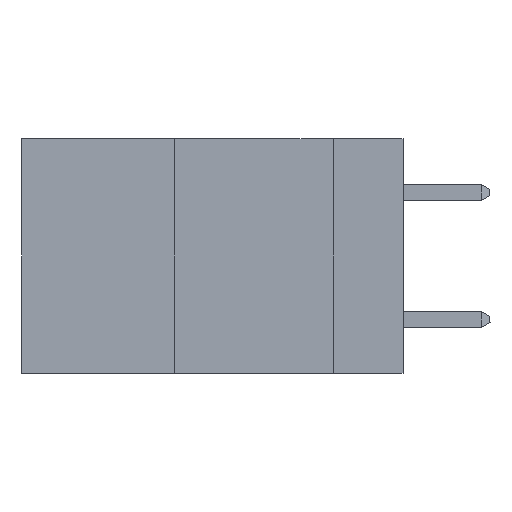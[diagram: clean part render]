
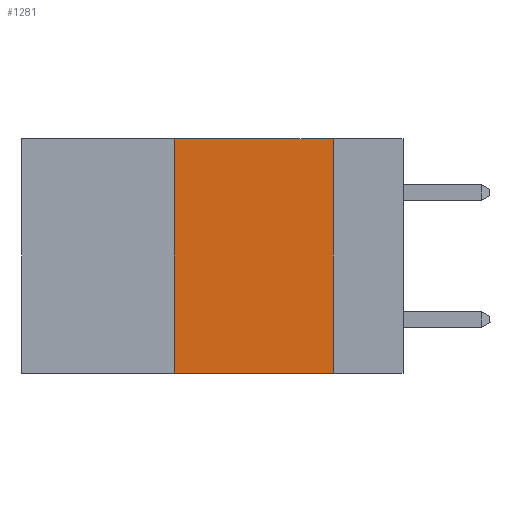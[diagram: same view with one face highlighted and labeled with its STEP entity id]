
A CAD part, left-side view. The second image highlights one B-rep face of the part: STEP entity #1281.
In plain terms, the highlighted planar face has unit normal (-1, 0, 0).
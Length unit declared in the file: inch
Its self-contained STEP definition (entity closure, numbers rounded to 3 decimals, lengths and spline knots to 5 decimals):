
#182 = CARTESIAN_POINT ( 'NONE',  ( 0., 0.11, -0.37 ) ) ;
#314 = DIRECTION ( 'NONE',  ( 0., -1., 0. ) ) ;
#464 = VERTEX_POINT ( 'NONE', #15426 ) ;
#518 = VECTOR ( 'NONE', #14986, 39.37008 ) ;
#656 = FACE_OUTER_BOUND ( 'NONE', #2852, .T. ) ;
#858 = AXIS2_PLACEMENT_3D ( 'NONE', #4481, #3514, #11802 ) ;
#1281 = ADVANCED_FACE ( 'NONE', ( #656 ), #10630, .F. ) ;
#2833 = VERTEX_POINT ( 'NONE', #182 ) ;
#2852 = EDGE_LOOP ( 'NONE', ( #10899, #14367, #5360, #5724 ) ) ;
#3158 = CARTESIAN_POINT ( 'NONE',  ( 0., 0.6, 0. ) ) ;
#3514 = DIRECTION ( 'NONE',  ( 1., 0., 0. ) ) ;
#4474 = EDGE_CURVE ( 'NONE', #464, #9095, #7384, .T. ) ;
#4481 = CARTESIAN_POINT ( 'NONE',  ( 0., 0.6, 0. ) ) ;
#4850 = CARTESIAN_POINT ( 'NONE',  ( 0., 0.36, -0.37 ) ) ;
#5073 = LINE ( 'NONE', #11168, #7831 ) ;
#5360 = ORIENTED_EDGE ( 'NONE', *, *, #6308, .F. ) ;
#5724 = ORIENTED_EDGE ( 'NONE', *, *, #8978, .T. ) ;
#6308 = EDGE_CURVE ( 'NONE', #8228, #464, #13209, .T. ) ;
#6745 = CARTESIAN_POINT ( 'NONE',  ( 0., 0.36, 0. ) ) ;
#7384 = LINE ( 'NONE', #3158, #10164 ) ;
#7831 = VECTOR ( 'NONE', #314, 39.37008 ) ;
#8228 = VERTEX_POINT ( 'NONE', #4850 ) ;
#8978 = EDGE_CURVE ( 'NONE', #8228, #2833, #5073, .T. ) ;
#9006 = CARTESIAN_POINT ( 'NONE',  ( 0., 0.11, 0. ) ) ;
#9072 = CARTESIAN_POINT ( 'NONE',  ( 0., 0.11, 0. ) ) ;
#9095 = VERTEX_POINT ( 'NONE', #9006 ) ;
#10164 = VECTOR ( 'NONE', #12644, 39.37008 ) ;
#10251 = DIRECTION ( 'NONE',  ( 0., 0., -1. ) ) ;
#10630 = PLANE ( 'NONE',  #858 ) ;
#10899 = ORIENTED_EDGE ( 'NONE', *, *, #15437, .F. ) ;
#11168 = CARTESIAN_POINT ( 'NONE',  ( 0., 0.6, -0.37 ) ) ;
#11802 = DIRECTION ( 'NONE',  ( 0., 0., -1. ) ) ;
#12587 = VECTOR ( 'NONE', #10251, 39.37008 ) ;
#12644 = DIRECTION ( 'NONE',  ( 0., -1., 0. ) ) ;
#12935 = LINE ( 'NONE', #9072, #12587 ) ;
#13209 = LINE ( 'NONE', #6745, #518 ) ;
#14367 = ORIENTED_EDGE ( 'NONE', *, *, #4474, .F. ) ;
#14986 = DIRECTION ( 'NONE',  ( 0., 0., 1. ) ) ;
#15426 = CARTESIAN_POINT ( 'NONE',  ( 0., 0.36, 0. ) ) ;
#15437 = EDGE_CURVE ( 'NONE', #9095, #2833, #12935, .T. ) ;
